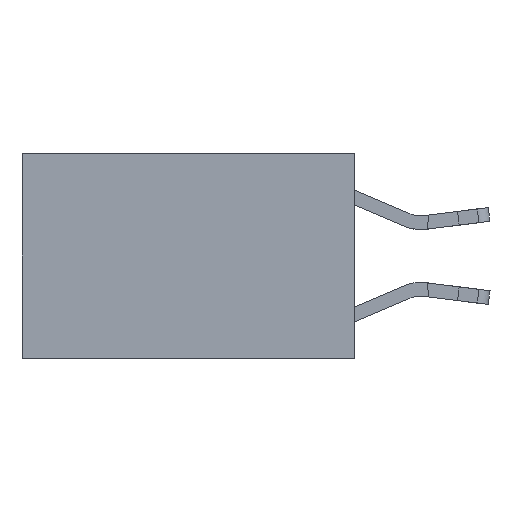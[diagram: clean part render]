
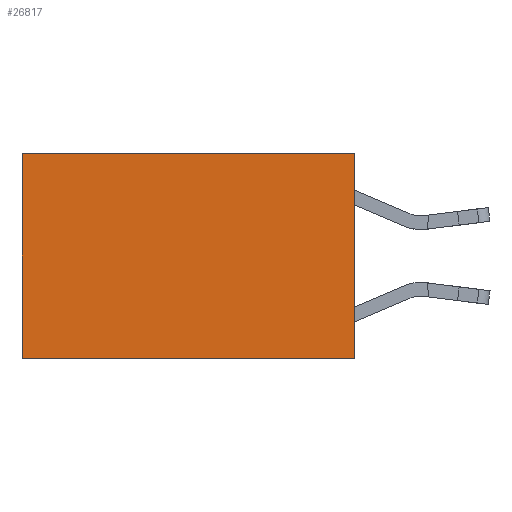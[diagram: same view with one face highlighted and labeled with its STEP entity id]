
A CAD part, left-side view. The second image highlights one B-rep face of the part: STEP entity #26817.
In plain terms, the highlighted planar face has unit normal (-1, 0, 0).
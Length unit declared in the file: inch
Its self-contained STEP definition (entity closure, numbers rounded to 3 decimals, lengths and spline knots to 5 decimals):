
#698 = VECTOR ( 'NONE', #3127, 39.37008 ) ;
#3124 = LINE ( 'NONE', #5191, #13500 ) ;
#3127 = DIRECTION ( 'NONE',  ( 0., 1., 0. ) ) ;
#3307 = LINE ( 'NONE', #23622, #698 ) ;
#3341 = AXIS2_PLACEMENT_3D ( 'NONE', #14596, #8143, #24820 ) ;
#3462 = FACE_OUTER_BOUND ( 'NONE', #12141, .T. ) ;
#3883 = PLANE ( 'NONE',  #3341 ) ;
#4704 = CARTESIAN_POINT ( 'NONE',  ( 0.2625, 0., -0.37 ) ) ;
#5057 = VERTEX_POINT ( 'NONE', #23075 ) ;
#5191 = CARTESIAN_POINT ( 'NONE',  ( 0.2625, 0., 0. ) ) ;
#5329 = ORIENTED_EDGE ( 'NONE', *, *, #7032, .T. ) ;
#7032 = EDGE_CURVE ( 'NONE', #25234, #9003, #3124, .T. ) ;
#7191 = CARTESIAN_POINT ( 'NONE',  ( 0.2625, 0., 0. ) ) ;
#7387 = DIRECTION ( 'NONE',  ( 0., 1., 0. ) ) ;
#7410 = VECTOR ( 'NONE', #24529, 39.37008 ) ;
#8143 = DIRECTION ( 'NONE',  ( 1., 0., 0. ) ) ;
#9003 = VERTEX_POINT ( 'NONE', #12251 ) ;
#9176 = VECTOR ( 'NONE', #22125, 39.37008 ) ;
#11243 = ORIENTED_EDGE ( 'NONE', *, *, #12216, .T. ) ;
#11704 = EDGE_CURVE ( 'NONE', #13677, #5057, #3307, .T. ) ;
#12141 = EDGE_LOOP ( 'NONE', ( #11243, #22252, #17488, #5329 ) ) ;
#12216 = EDGE_CURVE ( 'NONE', #9003, #5057, #25439, .T. ) ;
#12251 = CARTESIAN_POINT ( 'NONE',  ( 0.2625, 0.6, 0. ) ) ;
#13500 = VECTOR ( 'NONE', #7387, 39.37008 ) ;
#13677 = VERTEX_POINT ( 'NONE', #4704 ) ;
#14596 = CARTESIAN_POINT ( 'NONE',  ( 0.2625, 0., 0. ) ) ;
#17488 = ORIENTED_EDGE ( 'NONE', *, *, #21285, .F. ) ;
#18548 = LINE ( 'NONE', #24615, #7410 ) ;
#20140 = CARTESIAN_POINT ( 'NONE',  ( 0.2625, 0.6, 0. ) ) ;
#21285 = EDGE_CURVE ( 'NONE', #25234, #13677, #18548, .T. ) ;
#22125 = DIRECTION ( 'NONE',  ( 0., 0., -1. ) ) ;
#22252 = ORIENTED_EDGE ( 'NONE', *, *, #11704, .F. ) ;
#23075 = CARTESIAN_POINT ( 'NONE',  ( 0.2625, 0.6, -0.37 ) ) ;
#23622 = CARTESIAN_POINT ( 'NONE',  ( 0.2625, 0., -0.37 ) ) ;
#24529 = DIRECTION ( 'NONE',  ( 0., 0., -1. ) ) ;
#24615 = CARTESIAN_POINT ( 'NONE',  ( 0.2625, 0., 0. ) ) ;
#24820 = DIRECTION ( 'NONE',  ( 0., 0., -1. ) ) ;
#25234 = VERTEX_POINT ( 'NONE', #7191 ) ;
#25439 = LINE ( 'NONE', #20140, #9176 ) ;
#26817 = ADVANCED_FACE ( 'NONE', ( #3462 ), #3883, .F. ) ;
